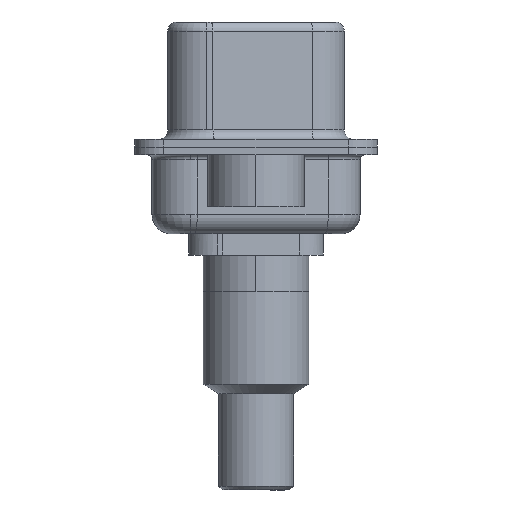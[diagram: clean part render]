
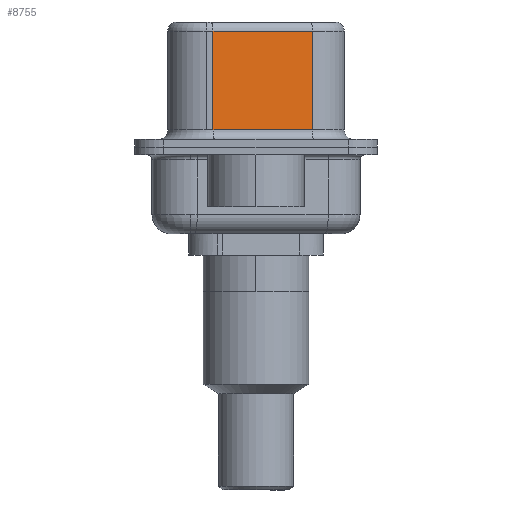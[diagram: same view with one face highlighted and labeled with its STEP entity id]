
A CAD part, left-side view. The second image highlights one B-rep face of the part: STEP entity #8755.
In plain terms, the highlighted planar face has unit normal (-0.985, -0.174, 0).
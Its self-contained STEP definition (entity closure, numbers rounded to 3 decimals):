
#368 = CARTESIAN_POINT ( 'NONE',  ( 4.585, -2.927, 0.9 ) ) ;
#1986 = CARTESIAN_POINT ( 'NONE',  ( 3.675, 2.233, 6.02 ) ) ;
#2423 = EDGE_CURVE ( 'NONE', #12657, #14597, #9543, .T. ) ;
#2884 = VECTOR ( 'NONE', #4481, 1000. ) ;
#3452 = AXIS2_PLACEMENT_3D ( 'NONE', #13054, #10266, #15686 ) ;
#3489 = FACE_OUTER_BOUND ( 'NONE', #17047, .T. ) ;
#4481 = DIRECTION ( 'NONE',  ( 0., 0., -1. ) ) ;
#5866 = LINE ( 'NONE', #7024, #12648 ) ;
#6527 = LINE ( 'NONE', #7138, #2884 ) ;
#6777 = VERTEX_POINT ( 'NONE', #7478 ) ;
#6878 = ORIENTED_EDGE ( 'NONE', *, *, #7623, .T. ) ;
#6882 = ORIENTED_EDGE ( 'NONE', *, *, #7542, .F. ) ;
#7024 = CARTESIAN_POINT ( 'NONE',  ( 4.585, -2.927, 6.02 ) ) ;
#7138 = CARTESIAN_POINT ( 'NONE',  ( 4.585, -2.927, 6.52 ) ) ;
#7341 = LINE ( 'NONE', #368, #12908 ) ;
#7478 = CARTESIAN_POINT ( 'NONE',  ( 4.585, -2.927, 6.02 ) ) ;
#7542 = EDGE_CURVE ( 'NONE', #6777, #13215, #6527, .T. ) ;
#7623 = EDGE_CURVE ( 'NONE', #14597, #13215, #7341, .T. ) ;
#7763 = CARTESIAN_POINT ( 'NONE',  ( 4.585, -2.927, 0.9 ) ) ;
#7916 = DIRECTION ( 'NONE',  ( 0., 0., -1. ) ) ;
#8359 = DIRECTION ( 'NONE',  ( -0.174, 0.985, 0. ) ) ;
#8585 = DIRECTION ( 'NONE',  ( 0.174, -0.985, 0. ) ) ;
#8755 = ADVANCED_FACE ( 'NONE', ( #3489 ), #14376, .F. ) ;
#9543 = LINE ( 'NONE', #11378, #12823 ) ;
#10266 = DIRECTION ( 'NONE',  ( 0.985, 0.174, 0. ) ) ;
#11378 = CARTESIAN_POINT ( 'NONE',  ( 3.675, 2.233, 6.52 ) ) ;
#11770 = ORIENTED_EDGE ( 'NONE', *, *, #2423, .T. ) ;
#12648 = VECTOR ( 'NONE', #8359, 1000. ) ;
#12657 = VERTEX_POINT ( 'NONE', #1986 ) ;
#12823 = VECTOR ( 'NONE', #7916, 1000. ) ;
#12908 = VECTOR ( 'NONE', #8585, 1000. ) ;
#13054 = CARTESIAN_POINT ( 'NONE',  ( 4.585, -2.927, 6.52 ) ) ;
#13215 = VERTEX_POINT ( 'NONE', #7763 ) ;
#13608 = EDGE_CURVE ( 'NONE', #6777, #12657, #5866, .T. ) ;
#14376 = PLANE ( 'NONE',  #3452 ) ;
#14597 = VERTEX_POINT ( 'NONE', #15631 ) ;
#15631 = CARTESIAN_POINT ( 'NONE',  ( 3.675, 2.233, 0.9 ) ) ;
#15686 = DIRECTION ( 'NONE',  ( -0.174, 0.985, 0. ) ) ;
#16505 = ORIENTED_EDGE ( 'NONE', *, *, #13608, .T. ) ;
#17047 = EDGE_LOOP ( 'NONE', ( #6882, #16505, #11770, #6878 ) ) ;
